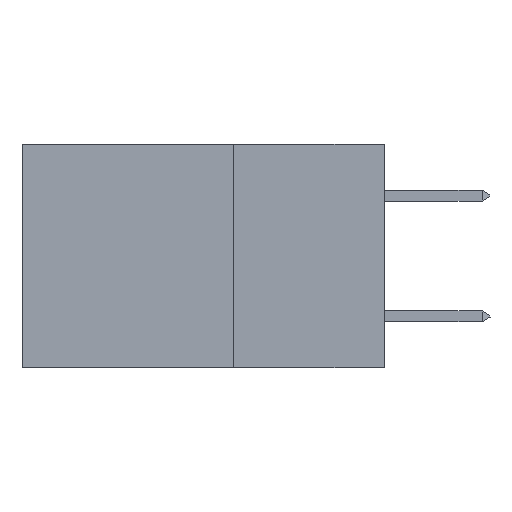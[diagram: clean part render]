
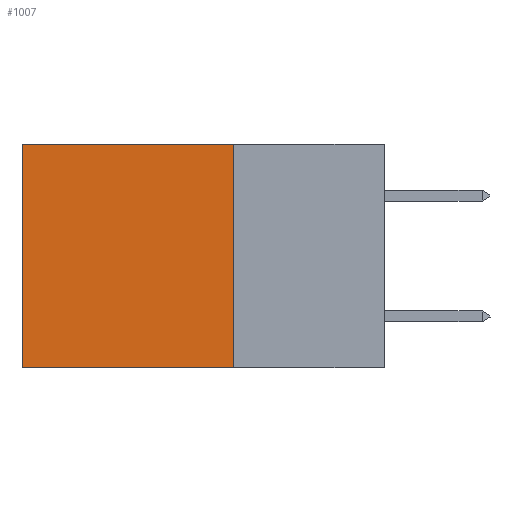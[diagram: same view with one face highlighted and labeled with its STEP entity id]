
A CAD part, left-side view. The second image highlights one B-rep face of the part: STEP entity #1007.
In plain terms, the highlighted planar face has unit normal (-1, 0, 0).
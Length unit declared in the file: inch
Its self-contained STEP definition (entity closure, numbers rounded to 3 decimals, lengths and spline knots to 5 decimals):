
#35 = LINE ( 'NONE', #13022, #2942 ) ;
#1007 = ADVANCED_FACE ( 'NONE', ( #29349 ), #30020, .F. ) ;
#2942 = VECTOR ( 'NONE', #29231, 39.37008 ) ;
#3057 = LINE ( 'NONE', #4116, #5646 ) ;
#3283 = ORIENTED_EDGE ( 'NONE', *, *, #20650, .F. ) ;
#4116 = CARTESIAN_POINT ( 'NONE',  ( 0.2875, 0.25, -0.37 ) ) ;
#4425 = CARTESIAN_POINT ( 'NONE',  ( 0.2875, 0.6, 0. ) ) ;
#5646 = VECTOR ( 'NONE', #24922, 39.37008 ) ;
#5903 = ORIENTED_EDGE ( 'NONE', *, *, #22527, .F. ) ;
#6052 = VECTOR ( 'NONE', #27620, 39.37008 ) ;
#7608 = ORIENTED_EDGE ( 'NONE', *, *, #20726, .T. ) ;
#7665 = VERTEX_POINT ( 'NONE', #27306 ) ;
#7683 = VECTOR ( 'NONE', #15887, 39.37008 ) ;
#9198 = DIRECTION ( 'NONE',  ( 0., 0., -1. ) ) ;
#11334 = EDGE_LOOP ( 'NONE', ( #17435, #3283, #5903, #7608 ) ) ;
#12612 = CARTESIAN_POINT ( 'NONE',  ( 0.2875, 0.25, 0. ) ) ;
#13022 = CARTESIAN_POINT ( 'NONE',  ( 0.2875, 0.25, 0. ) ) ;
#15603 = VERTEX_POINT ( 'NONE', #12612 ) ;
#15874 = LINE ( 'NONE', #25134, #6052 ) ;
#15887 = DIRECTION ( 'NONE',  ( 0., 0., -1. ) ) ;
#16837 = EDGE_CURVE ( 'NONE', #22522, #21635, #26380, .T. ) ;
#17435 = ORIENTED_EDGE ( 'NONE', *, *, #16837, .T. ) ;
#17695 = CARTESIAN_POINT ( 'NONE',  ( 0.2875, 0.6, 0. ) ) ;
#20650 = EDGE_CURVE ( 'NONE', #7665, #21635, #3057, .T. ) ;
#20726 = EDGE_CURVE ( 'NONE', #15603, #22522, #15874, .T. ) ;
#21635 = VERTEX_POINT ( 'NONE', #30076 ) ;
#22522 = VERTEX_POINT ( 'NONE', #17695 ) ;
#22527 = EDGE_CURVE ( 'NONE', #15603, #7665, #35, .T. ) ;
#24184 = AXIS2_PLACEMENT_3D ( 'NONE', #27979, #27874, #9198 ) ;
#24922 = DIRECTION ( 'NONE',  ( 0., 1., 0. ) ) ;
#25134 = CARTESIAN_POINT ( 'NONE',  ( 0.2875, 0.25, 0. ) ) ;
#26380 = LINE ( 'NONE', #4425, #7683 ) ;
#27306 = CARTESIAN_POINT ( 'NONE',  ( 0.2875, 0.25, -0.37 ) ) ;
#27620 = DIRECTION ( 'NONE',  ( 0., 1., 0. ) ) ;
#27874 = DIRECTION ( 'NONE',  ( 1., 0., 0. ) ) ;
#27979 = CARTESIAN_POINT ( 'NONE',  ( 0.2875, 0.25, 0. ) ) ;
#29231 = DIRECTION ( 'NONE',  ( 0., 0., -1. ) ) ;
#29349 = FACE_OUTER_BOUND ( 'NONE', #11334, .T. ) ;
#30020 = PLANE ( 'NONE',  #24184 ) ;
#30076 = CARTESIAN_POINT ( 'NONE',  ( 0.2875, 0.6, -0.37 ) ) ;
